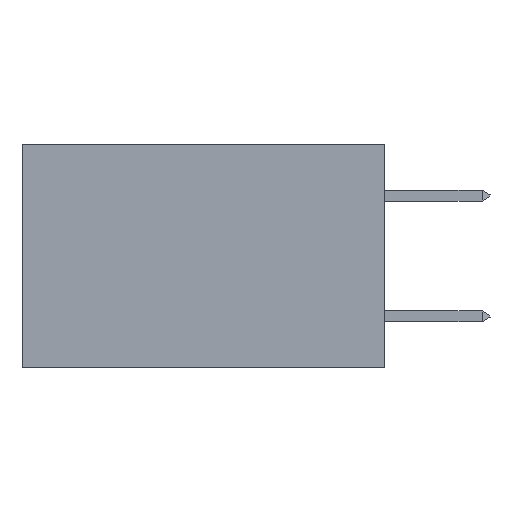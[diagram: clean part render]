
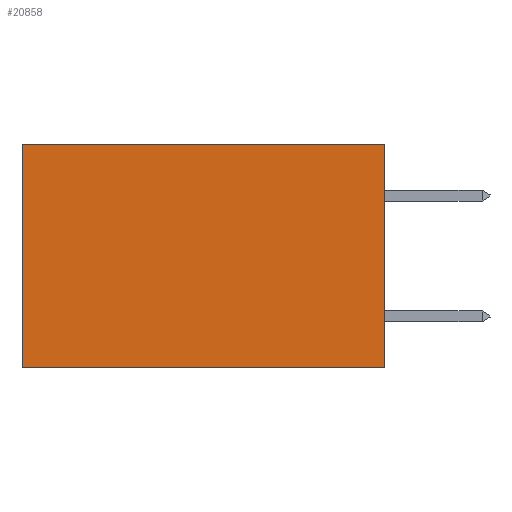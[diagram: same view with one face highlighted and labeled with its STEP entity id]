
A CAD part, left-side view. The second image highlights one B-rep face of the part: STEP entity #20858.
In plain terms, the highlighted planar face has unit normal (-1, 0, 0).
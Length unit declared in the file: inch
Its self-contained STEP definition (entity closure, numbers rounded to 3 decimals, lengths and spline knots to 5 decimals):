
#674 = CARTESIAN_POINT ( 'NONE',  ( 0.2875, 0.6, 0. ) ) ;
#1666 = CARTESIAN_POINT ( 'NONE',  ( 0.2875, 0., -0.37 ) ) ;
#2066 = EDGE_LOOP ( 'NONE', ( #35391, #7298, #36756, #12518 ) ) ;
#3070 = DIRECTION ( 'NONE',  ( 0., 1., 0. ) ) ;
#3150 = VERTEX_POINT ( 'NONE', #16635 ) ;
#3611 = EDGE_CURVE ( 'NONE', #15633, #7742, #17579, .T. ) ;
#4089 = VECTOR ( 'NONE', #31029, 39.37008 ) ;
#5385 = CARTESIAN_POINT ( 'NONE',  ( 0.2875, 0., 0. ) ) ;
#6007 = LINE ( 'NONE', #25267, #4089 ) ;
#7298 = ORIENTED_EDGE ( 'NONE', *, *, #3611, .F. ) ;
#7742 = VERTEX_POINT ( 'NONE', #17010 ) ;
#8431 = DIRECTION ( 'NONE',  ( 0., 0., -1. ) ) ;
#9836 = CARTESIAN_POINT ( 'NONE',  ( 0.2875, 0.6, 0. ) ) ;
#10751 = AXIS2_PLACEMENT_3D ( 'NONE', #5385, #26343, #8431 ) ;
#10830 = LINE ( 'NONE', #9836, #33579 ) ;
#12518 = ORIENTED_EDGE ( 'NONE', *, *, #27149, .T. ) ;
#15633 = VERTEX_POINT ( 'NONE', #1666 ) ;
#16635 = CARTESIAN_POINT ( 'NONE',  ( 0.2875, 0., 0. ) ) ;
#16968 = FACE_OUTER_BOUND ( 'NONE', #2066, .T. ) ;
#17010 = CARTESIAN_POINT ( 'NONE',  ( 0.2875, 0.6, -0.37 ) ) ;
#17579 = LINE ( 'NONE', #21550, #25497 ) ;
#19167 = EDGE_CURVE ( 'NONE', #32376, #7742, #10830, .T. ) ;
#20374 = PLANE ( 'NONE',  #10751 ) ;
#20858 = ADVANCED_FACE ( 'NONE', ( #16968 ), #20374, .F. ) ;
#21106 = CARTESIAN_POINT ( 'NONE',  ( 0.2875, 0., 0. ) ) ;
#21550 = CARTESIAN_POINT ( 'NONE',  ( 0.2875, 0., -0.37 ) ) ;
#25267 = CARTESIAN_POINT ( 'NONE',  ( 0.2875, 0., 0. ) ) ;
#25497 = VECTOR ( 'NONE', #36231, 39.37008 ) ;
#26343 = DIRECTION ( 'NONE',  ( 1., 0., 0. ) ) ;
#27149 = EDGE_CURVE ( 'NONE', #3150, #32376, #38395, .T. ) ;
#27678 = DIRECTION ( 'NONE',  ( 0., 0., -1. ) ) ;
#30554 = VECTOR ( 'NONE', #3070, 39.37008 ) ;
#31029 = DIRECTION ( 'NONE',  ( 0., 0., -1. ) ) ;
#32376 = VERTEX_POINT ( 'NONE', #674 ) ;
#33579 = VECTOR ( 'NONE', #27678, 39.37008 ) ;
#35391 = ORIENTED_EDGE ( 'NONE', *, *, #19167, .T. ) ;
#36153 = EDGE_CURVE ( 'NONE', #3150, #15633, #6007, .T. ) ;
#36231 = DIRECTION ( 'NONE',  ( 0., 1., 0. ) ) ;
#36756 = ORIENTED_EDGE ( 'NONE', *, *, #36153, .F. ) ;
#38395 = LINE ( 'NONE', #21106, #30554 ) ;
